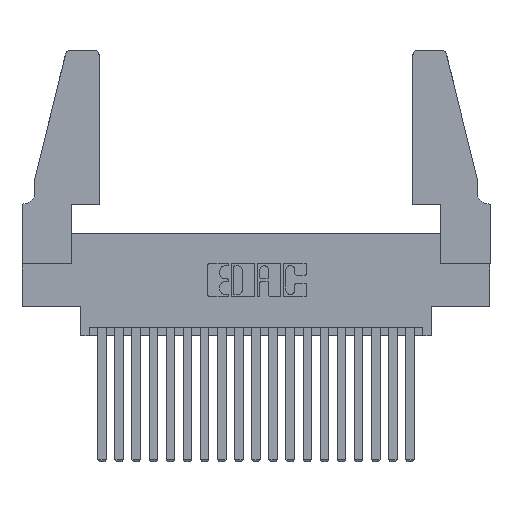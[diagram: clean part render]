
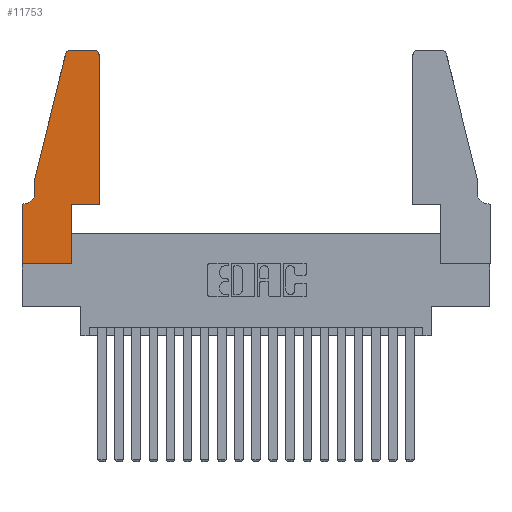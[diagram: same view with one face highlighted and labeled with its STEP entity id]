
A CAD part, top view. The second image highlights one B-rep face of the part: STEP entity #11753.
In plain terms, the highlighted planar face has unit normal (0, 0, 1).
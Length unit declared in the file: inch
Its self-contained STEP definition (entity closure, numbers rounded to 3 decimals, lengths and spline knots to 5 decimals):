
#727 = ORIENTED_EDGE ( 'NONE', *, *, #4626, .T. ) ;
#1348 = DIRECTION ( 'NONE',  ( 0., -1., 0. ) ) ;
#1371 = CARTESIAN_POINT ( 'NONE',  ( 0.4505, 0.35, 0.37 ) ) ;
#1400 = DIRECTION ( 'NONE',  ( 1., 0., 0. ) ) ;
#1472 = DIRECTION ( 'NONE',  ( 1., 0., 0. ) ) ;
#1517 = AXIS2_PLACEMENT_3D ( 'NONE', #6548, #8140, #18894 ) ;
#1642 = CARTESIAN_POINT ( 'NONE',  ( 0.2865, 0.35, 0.37 ) ) ;
#1897 = ORIENTED_EDGE ( 'NONE', *, *, #14793, .T. ) ;
#2658 = VECTOR ( 'NONE', #3685, 39.37008 ) ;
#2728 = VERTEX_POINT ( 'NONE', #19271 ) ;
#3215 = FACE_OUTER_BOUND ( 'NONE', #8040, .T. ) ;
#3361 = CARTESIAN_POINT ( 'NONE',  ( 0.2865, 0.35, 0.37 ) ) ;
#3382 = DIRECTION ( 'NONE',  ( 0., 0., 1. ) ) ;
#3685 = DIRECTION ( 'NONE',  ( 0., -1., 0. ) ) ;
#3739 = DIRECTION ( 'NONE',  ( -1., 0., 0. ) ) ;
#3813 = LINE ( 'NONE', #16875, #19672 ) ;
#4010 = DIRECTION ( 'NONE',  ( 0., 1., 0. ) ) ;
#4282 = VECTOR ( 'NONE', #20025, 39.37008 ) ;
#4491 = EDGE_CURVE ( 'NONE', #19955, #14694, #5264, .T. ) ;
#4626 = EDGE_CURVE ( 'NONE', #6389, #9607, #7938, .T. ) ;
#5028 = EDGE_CURVE ( 'NONE', #9881, #6806, #3813, .T. ) ;
#5179 = CARTESIAN_POINT ( 'NONE',  ( 0.0755, 0.5, 0.37 ) ) ;
#5264 = LINE ( 'NONE', #13036, #18058 ) ;
#5332 = CARTESIAN_POINT ( 'NONE',  ( 0.25487, 1.22718, 0.37 ) ) ;
#5602 = AXIS2_PLACEMENT_3D ( 'NONE', #19938, #10810, #1400 ) ;
#5721 = CARTESIAN_POINT ( 'NONE',  ( 0.0055, 0.35, 0.37 ) ) ;
#5767 = VECTOR ( 'NONE', #9848, 39.37008 ) ;
#5796 = CARTESIAN_POINT ( 'NONE',  ( 0.0755, 0.42, 0.37 ) ) ;
#6151 = ORIENTED_EDGE ( 'NONE', *, *, #7649, .T. ) ;
#6389 = VERTEX_POINT ( 'NONE', #1371 ) ;
#6489 = EDGE_CURVE ( 'NONE', #14466, #6389, #11786, .T. ) ;
#6548 = CARTESIAN_POINT ( 'NONE',  ( 0., 0.35, 0.37 ) ) ;
#6583 = VERTEX_POINT ( 'NONE', #5332 ) ;
#6806 = VERTEX_POINT ( 'NONE', #5796 ) ;
#6941 = VECTOR ( 'NONE', #4010, 39.37008 ) ;
#7184 = DIRECTION ( 'NONE',  ( 0., 0., -1. ) ) ;
#7513 = CARTESIAN_POINT ( 'NONE',  ( 0.0755, 0.5, 0.37 ) ) ;
#7649 = EDGE_CURVE ( 'NONE', #9607, #19955, #7830, .T. ) ;
#7760 = CARTESIAN_POINT ( 'NONE',  ( 0.0755, 0.35, 0.37 ) ) ;
#7830 = CIRCLE ( 'NONE', #5602, 0.03 ) ;
#7863 = LINE ( 'NONE', #3361, #8359 ) ;
#7938 = LINE ( 'NONE', #10169, #6941 ) ;
#8040 = EDGE_LOOP ( 'NONE', ( #18440, #8956, #14161, #16887, #1897, #9092, #15072, #8519, #11631, #12707, #727, #6151 ) ) ;
#8140 = DIRECTION ( 'NONE',  ( 0., 0., 1. ) ) ;
#8359 = VECTOR ( 'NONE', #15766, 39.37008 ) ;
#8417 = CARTESIAN_POINT ( 'NONE',  ( 0.4505, 1.22, 0.37 ) ) ;
#8519 = ORIENTED_EDGE ( 'NONE', *, *, #9354, .T. ) ;
#8956 = ORIENTED_EDGE ( 'NONE', *, *, #10090, .T. ) ;
#9092 = ORIENTED_EDGE ( 'NONE', *, *, #16196, .T. ) ;
#9346 = LINE ( 'NONE', #7760, #4282 ) ;
#9354 = EDGE_CURVE ( 'NONE', #10708, #14949, #17638, .T. ) ;
#9565 = EDGE_CURVE ( 'NONE', #2728, #10708, #15061, .T. ) ;
#9607 = VERTEX_POINT ( 'NONE', #8417 ) ;
#9848 = DIRECTION ( 'NONE',  ( -0.239, -0.971, 0. ) ) ;
#9881 = VERTEX_POINT ( 'NONE', #7513 ) ;
#9893 = LINE ( 'NONE', #5179, #5767 ) ;
#10090 = EDGE_CURVE ( 'NONE', #14694, #6583, #18572, .T. ) ;
#10169 = CARTESIAN_POINT ( 'NONE',  ( 0.4505, 0.35, 0.37 ) ) ;
#10499 = VERTEX_POINT ( 'NONE', #5721 ) ;
#10708 = VERTEX_POINT ( 'NONE', #17070 ) ;
#10810 = DIRECTION ( 'NONE',  ( 0., 0., 1. ) ) ;
#11348 = CARTESIAN_POINT ( 'NONE',  ( 0.4505, 0.35, 0.37 ) ) ;
#11631 = ORIENTED_EDGE ( 'NONE', *, *, #17163, .T. ) ;
#11753 = ADVANCED_FACE ( 'NONE', ( #3215 ), #17375, .T. ) ;
#11758 = CARTESIAN_POINT ( 'NONE',  ( 0.4205, 1.25, 0.37 ) ) ;
#11786 = LINE ( 'NONE', #11348, #14927 ) ;
#12433 = CARTESIAN_POINT ( 'NONE',  ( 0., 0., 0.37 ) ) ;
#12688 = CARTESIAN_POINT ( 'NONE',  ( 0.284, 1.22, 0.37 ) ) ;
#12707 = ORIENTED_EDGE ( 'NONE', *, *, #6489, .T. ) ;
#13036 = CARTESIAN_POINT ( 'NONE',  ( 0.2605, 1.25, 0.37 ) ) ;
#13595 = VECTOR ( 'NONE', #1472, 39.37008 ) ;
#13731 = CARTESIAN_POINT ( 'NONE',  ( 0.2865, 0., 0.37 ) ) ;
#14035 = AXIS2_PLACEMENT_3D ( 'NONE', #16456, #7184, #17979 ) ;
#14161 = ORIENTED_EDGE ( 'NONE', *, *, #19127, .T. ) ;
#14239 = DIRECTION ( 'NONE',  ( 1., 0., 0. ) ) ;
#14255 = CIRCLE ( 'NONE', #14035, 0.07 ) ;
#14466 = VERTEX_POINT ( 'NONE', #1642 ) ;
#14540 = CARTESIAN_POINT ( 'NONE',  ( 0., 0., 0.37 ) ) ;
#14694 = VERTEX_POINT ( 'NONE', #19174 ) ;
#14793 = EDGE_CURVE ( 'NONE', #6806, #10499, #14255, .T. ) ;
#14927 = VECTOR ( 'NONE', #15981, 39.37008 ) ;
#14949 = VERTEX_POINT ( 'NONE', #13731 ) ;
#15061 = LINE ( 'NONE', #14540, #2658 ) ;
#15072 = ORIENTED_EDGE ( 'NONE', *, *, #9565, .T. ) ;
#15766 = DIRECTION ( 'NONE',  ( 0., 1., 0. ) ) ;
#15981 = DIRECTION ( 'NONE',  ( 1., 0., 0. ) ) ;
#16196 = EDGE_CURVE ( 'NONE', #10499, #2728, #9346, .T. ) ;
#16456 = CARTESIAN_POINT ( 'NONE',  ( 0.0055, 0.42, 0.37 ) ) ;
#16875 = CARTESIAN_POINT ( 'NONE',  ( 0.0755, 0.5, 0.37 ) ) ;
#16887 = ORIENTED_EDGE ( 'NONE', *, *, #5028, .T. ) ;
#17070 = CARTESIAN_POINT ( 'NONE',  ( 0., 0., 0.37 ) ) ;
#17163 = EDGE_CURVE ( 'NONE', #14949, #14466, #7863, .T. ) ;
#17375 = PLANE ( 'NONE',  #1517 ) ;
#17638 = LINE ( 'NONE', #12433, #13595 ) ;
#17979 = DIRECTION ( 'NONE',  ( -1., 0., 0. ) ) ;
#18058 = VECTOR ( 'NONE', #3739, 39.37008 ) ;
#18394 = AXIS2_PLACEMENT_3D ( 'NONE', #12688, #3382, #14239 ) ;
#18440 = ORIENTED_EDGE ( 'NONE', *, *, #4491, .T. ) ;
#18572 = CIRCLE ( 'NONE', #18394, 0.03 ) ;
#18894 = DIRECTION ( 'NONE',  ( 1., 0., 0. ) ) ;
#19127 = EDGE_CURVE ( 'NONE', #6583, #9881, #9893, .T. ) ;
#19174 = CARTESIAN_POINT ( 'NONE',  ( 0.284, 1.25, 0.37 ) ) ;
#19271 = CARTESIAN_POINT ( 'NONE',  ( 0., 0.35, 0.37 ) ) ;
#19672 = VECTOR ( 'NONE', #1348, 39.37008 ) ;
#19938 = CARTESIAN_POINT ( 'NONE',  ( 0.4205, 1.22, 0.37 ) ) ;
#19955 = VERTEX_POINT ( 'NONE', #11758 ) ;
#20025 = DIRECTION ( 'NONE',  ( -1., 0., 0. ) ) ;
